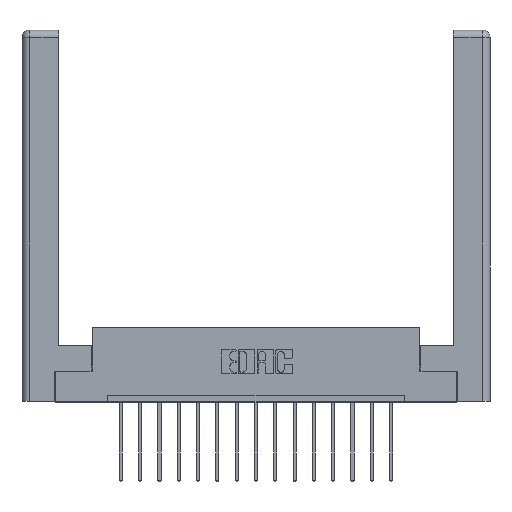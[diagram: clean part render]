
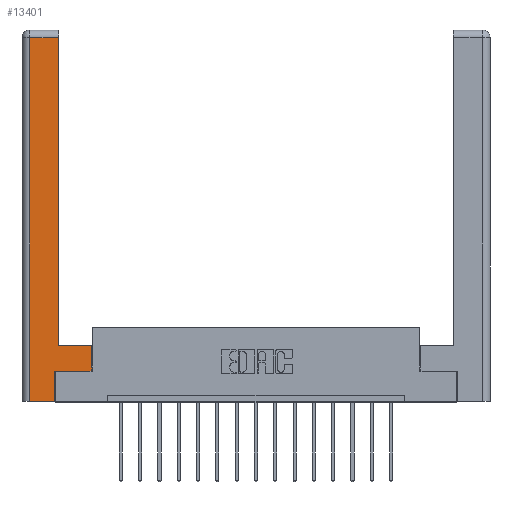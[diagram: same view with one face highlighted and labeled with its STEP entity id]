
A CAD part, top view. The second image highlights one B-rep face of the part: STEP entity #13401.
In plain terms, the highlighted planar face has unit normal (0, 0, 1).
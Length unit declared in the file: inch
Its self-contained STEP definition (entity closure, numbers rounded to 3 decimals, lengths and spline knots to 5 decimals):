
#395 = ORIENTED_EDGE ( 'NONE', *, *, #12436, .T. ) ;
#648 = VERTEX_POINT ( 'NONE', #8279 ) ;
#964 = CARTESIAN_POINT ( 'NONE',  ( 0.265, 0., 0. ) ) ;
#1843 = VECTOR ( 'NONE', #13076, 39.37008 ) ;
#1930 = CARTESIAN_POINT ( 'NONE',  ( 0.565, 0.45, 0. ) ) ;
#2100 = CARTESIAN_POINT ( 'NONE',  ( 0.295, 0.45, 0. ) ) ;
#2331 = FACE_OUTER_BOUND ( 'NONE', #11246, .T. ) ;
#2617 = VERTEX_POINT ( 'NONE', #7275 ) ;
#2686 = ORIENTED_EDGE ( 'NONE', *, *, #12410, .T. ) ;
#2965 = ORIENTED_EDGE ( 'NONE', *, *, #13760, .T. ) ;
#3427 = LINE ( 'NONE', #8328, #13709 ) ;
#3534 = CARTESIAN_POINT ( 'NONE',  ( 0.295, 2.94, 0. ) ) ;
#3552 = LINE ( 'NONE', #2100, #4387 ) ;
#3763 = CARTESIAN_POINT ( 'NONE',  ( 0.0615, 0., 0. ) ) ;
#4101 = VECTOR ( 'NONE', #16165, 39.37008 ) ;
#4160 = VERTEX_POINT ( 'NONE', #10354 ) ;
#4329 = EDGE_CURVE ( 'NONE', #2617, #9539, #16910, .T. ) ;
#4387 = VECTOR ( 'NONE', #12828, 39.37008 ) ;
#5171 = EDGE_CURVE ( 'NONE', #7639, #5675, #10207, .T. ) ;
#5369 = CARTESIAN_POINT ( 'NONE',  ( 0.265, 0., 0. ) ) ;
#5397 = DIRECTION ( 'NONE',  ( 0., 1., 0. ) ) ;
#5535 = ORIENTED_EDGE ( 'NONE', *, *, #4329, .T. ) ;
#5640 = LINE ( 'NONE', #1930, #17149 ) ;
#5675 = VERTEX_POINT ( 'NONE', #3534 ) ;
#5789 = VERTEX_POINT ( 'NONE', #964 ) ;
#5908 = DIRECTION ( 'NONE',  ( 0., 1., 0. ) ) ;
#6064 = VECTOR ( 'NONE', #14769, 39.37008 ) ;
#6493 = LINE ( 'NONE', #5369, #6064 ) ;
#6502 = PLANE ( 'NONE',  #16086 ) ;
#6810 = EDGE_CURVE ( 'NONE', #648, #17160, #17069, .T. ) ;
#7079 = CARTESIAN_POINT ( 'NONE',  ( 0.565, 0.245, 0. ) ) ;
#7275 = CARTESIAN_POINT ( 'NONE',  ( 0.265, 0.245, 0. ) ) ;
#7292 = ORIENTED_EDGE ( 'NONE', *, *, #7939, .T. ) ;
#7293 = CARTESIAN_POINT ( 'NONE',  ( 0.295, 0.45, 0. ) ) ;
#7639 = VERTEX_POINT ( 'NONE', #7293 ) ;
#7801 = CARTESIAN_POINT ( 'NONE',  ( 0., 0., 0. ) ) ;
#7939 = EDGE_CURVE ( 'NONE', #5675, #648, #3427, .T. ) ;
#8228 = EDGE_CURVE ( 'NONE', #5789, #2617, #13504, .T. ) ;
#8279 = CARTESIAN_POINT ( 'NONE',  ( 0.0615, 2.94, 0. ) ) ;
#8328 = CARTESIAN_POINT ( 'NONE',  ( 0.0615, 2.94, 0. ) ) ;
#9539 = VERTEX_POINT ( 'NONE', #7079 ) ;
#10207 = LINE ( 'NONE', #16064, #15851 ) ;
#10333 = CARTESIAN_POINT ( 'NONE',  ( 0.565, 0.245, 0. ) ) ;
#10354 = CARTESIAN_POINT ( 'NONE',  ( 0.565, 0.45, 0. ) ) ;
#10920 = CARTESIAN_POINT ( 'NONE',  ( 0.0615, 0., 0. ) ) ;
#11246 = EDGE_LOOP ( 'NONE', ( #17277, #7292, #16139, #2965, #12949, #5535, #395, #2686 ) ) ;
#11898 = DIRECTION ( 'NONE',  ( -1., 0., 0. ) ) ;
#12410 = EDGE_CURVE ( 'NONE', #4160, #7639, #3552, .T. ) ;
#12436 = EDGE_CURVE ( 'NONE', #9539, #4160, #5640, .T. ) ;
#12828 = DIRECTION ( 'NONE',  ( -1., 0., 0. ) ) ;
#12949 = ORIENTED_EDGE ( 'NONE', *, *, #8228, .T. ) ;
#13076 = DIRECTION ( 'NONE',  ( 1., 0., 0. ) ) ;
#13248 = DIRECTION ( 'NONE',  ( 0., 0., -1. ) ) ;
#13401 = ADVANCED_FACE ( 'NONE', ( #2331 ), #6502, .F. ) ;
#13504 = LINE ( 'NONE', #15448, #16428 ) ;
#13709 = VECTOR ( 'NONE', #15063, 39.37008 ) ;
#13760 = EDGE_CURVE ( 'NONE', #17160, #5789, #6493, .T. ) ;
#14769 = DIRECTION ( 'NONE',  ( 1., 0., 0. ) ) ;
#15063 = DIRECTION ( 'NONE',  ( -1., 0., 0. ) ) ;
#15448 = CARTESIAN_POINT ( 'NONE',  ( 0.265, 0.245, 0. ) ) ;
#15851 = VECTOR ( 'NONE', #5397, 39.37008 ) ;
#16064 = CARTESIAN_POINT ( 'NONE',  ( 0.295, 3., 0. ) ) ;
#16086 = AXIS2_PLACEMENT_3D ( 'NONE', #7801, #13248, #11898 ) ;
#16139 = ORIENTED_EDGE ( 'NONE', *, *, #6810, .T. ) ;
#16165 = DIRECTION ( 'NONE',  ( 0., -1., 0. ) ) ;
#16428 = VECTOR ( 'NONE', #16954, 39.37008 ) ;
#16910 = LINE ( 'NONE', #10333, #1843 ) ;
#16954 = DIRECTION ( 'NONE',  ( 0., 1., 0. ) ) ;
#17069 = LINE ( 'NONE', #10920, #4101 ) ;
#17149 = VECTOR ( 'NONE', #5908, 39.37008 ) ;
#17160 = VERTEX_POINT ( 'NONE', #3763 ) ;
#17277 = ORIENTED_EDGE ( 'NONE', *, *, #5171, .T. ) ;
